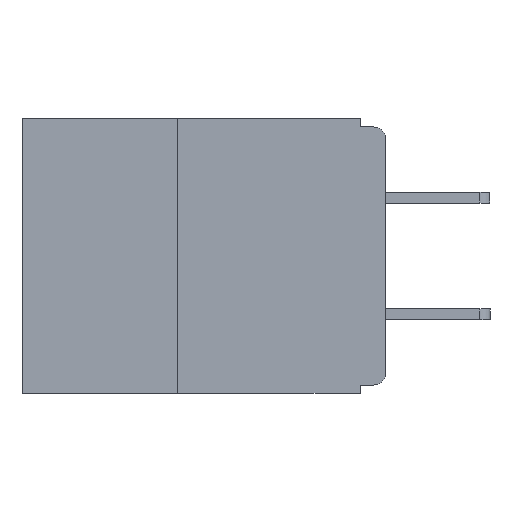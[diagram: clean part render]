
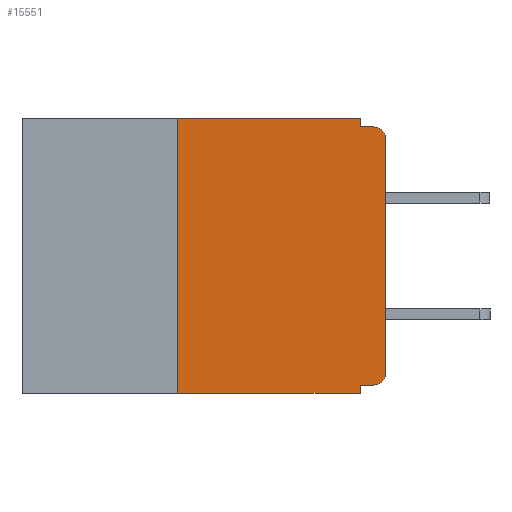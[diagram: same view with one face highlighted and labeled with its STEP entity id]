
A CAD part, left-side view. The second image highlights one B-rep face of the part: STEP entity #15551.
In plain terms, the highlighted planar face has unit normal (-1, 0, 0).
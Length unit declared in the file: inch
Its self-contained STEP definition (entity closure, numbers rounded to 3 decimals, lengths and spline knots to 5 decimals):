
#156 = LINE ( 'NONE', #7414, #13391 ) ;
#546 = CARTESIAN_POINT ( 'NONE',  ( 0., 0.437, 0. ) ) ;
#576 = ORIENTED_EDGE ( 'NONE', *, *, #13865, .F. ) ;
#692 = DIRECTION ( 'NONE',  ( 0., -1., 0. ) ) ;
#1141 = CARTESIAN_POINT ( 'NONE',  ( 0., 0.437, -0.33 ) ) ;
#1366 = CARTESIAN_POINT ( 'NONE',  ( 0., 0.031, 0. ) ) ;
#1687 = CARTESIAN_POINT ( 'NONE',  ( 0., 0.031, 0. ) ) ;
#1850 = VERTEX_POINT ( 'NONE', #1687 ) ;
#1886 = DIRECTION ( 'NONE',  ( 1., 0., 0. ) ) ;
#2242 = EDGE_CURVE ( 'NONE', #14894, #14790, #11142, .T. ) ;
#2300 = DIRECTION ( 'NONE',  ( 0., 0., 1. ) ) ;
#2543 = AXIS2_PLACEMENT_3D ( 'NONE', #3014, #3001, #2996 ) ;
#2635 = VERTEX_POINT ( 'NONE', #13340 ) ;
#2672 = CARTESIAN_POINT ( 'NONE',  ( 0., 0.015, -0.01 ) ) ;
#2711 = LINE ( 'NONE', #8479, #3135 ) ;
#2727 = VECTOR ( 'NONE', #15027, 39.37008 ) ;
#2996 = DIRECTION ( 'NONE',  ( 0., 0., -1. ) ) ;
#3001 = DIRECTION ( 'NONE',  ( -1., 0., 0. ) ) ;
#3014 = CARTESIAN_POINT ( 'NONE',  ( 0., 0.015, -0.025 ) ) ;
#3135 = VECTOR ( 'NONE', #3293, 39.37008 ) ;
#3293 = DIRECTION ( 'NONE',  ( 0., -1., 0. ) ) ;
#3350 = AXIS2_PLACEMENT_3D ( 'NONE', #13615, #15105, #15219 ) ;
#3510 = VECTOR ( 'NONE', #13485, 39.37008 ) ;
#4034 = AXIS2_PLACEMENT_3D ( 'NONE', #546, #1886, #10865 ) ;
#4115 = DIRECTION ( 'NONE',  ( 0., 0., -1. ) ) ;
#4569 = CIRCLE ( 'NONE', #2543, 0.015 ) ;
#5411 = EDGE_CURVE ( 'NONE', #15789, #10457, #12205, .T. ) ;
#5886 = LINE ( 'NONE', #14158, #15485 ) ;
#6221 = CARTESIAN_POINT ( 'NONE',  ( 0., 0.031, -0.33 ) ) ;
#6424 = CARTESIAN_POINT ( 'NONE',  ( 0., 0., -0.305 ) ) ;
#6653 = CARTESIAN_POINT ( 'NONE',  ( 0., 0.015, -0.32 ) ) ;
#6882 = LINE ( 'NONE', #10980, #3510 ) ;
#7287 = ORIENTED_EDGE ( 'NONE', *, *, #5411, .T. ) ;
#7289 = VECTOR ( 'NONE', #7389, 39.37008 ) ;
#7389 = DIRECTION ( 'NONE',  ( 0., 1., 0. ) ) ;
#7414 = CARTESIAN_POINT ( 'NONE',  ( 0., 0.25, -0.33 ) ) ;
#8040 = ORIENTED_EDGE ( 'NONE', *, *, #8428, .T. ) ;
#8296 = PLANE ( 'NONE',  #4034 ) ;
#8381 = CARTESIAN_POINT ( 'NONE',  ( 0., 0.031, -0.01 ) ) ;
#8394 = ORIENTED_EDGE ( 'NONE', *, *, #11517, .F. ) ;
#8428 = EDGE_CURVE ( 'NONE', #10171, #8513, #4569, .T. ) ;
#8479 = CARTESIAN_POINT ( 'NONE',  ( 0., 0.437, 0. ) ) ;
#8513 = VERTEX_POINT ( 'NONE', #2672 ) ;
#8784 = CARTESIAN_POINT ( 'NONE',  ( 0., 0., 0. ) ) ;
#8802 = EDGE_CURVE ( 'NONE', #1850, #9108, #15712, .T. ) ;
#8861 = CARTESIAN_POINT ( 'NONE',  ( 0., 0.25, -0.33 ) ) ;
#9108 = VERTEX_POINT ( 'NONE', #8381 ) ;
#9187 = EDGE_CURVE ( 'NONE', #14790, #10171, #12879, .T. ) ;
#9677 = EDGE_CURVE ( 'NONE', #15956, #1850, #2711, .T. ) ;
#10171 = VERTEX_POINT ( 'NONE', #14426 ) ;
#10397 = EDGE_CURVE ( 'NONE', #14894, #2635, #13982, .T. ) ;
#10457 = VERTEX_POINT ( 'NONE', #6221 ) ;
#10865 = DIRECTION ( 'NONE',  ( 0., 0., -1. ) ) ;
#10980 = CARTESIAN_POINT ( 'NONE',  ( 0., 0., -0.01 ) ) ;
#11142 = CIRCLE ( 'NONE', #3350, 0.015 ) ;
#11230 = FACE_OUTER_BOUND ( 'NONE', #11752, .T. ) ;
#11517 = EDGE_CURVE ( 'NONE', #9108, #8513, #6882, .T. ) ;
#11534 = ORIENTED_EDGE ( 'NONE', *, *, #11734, .F. ) ;
#11734 = EDGE_CURVE ( 'NONE', #15789, #15956, #156, .T. ) ;
#11752 = EDGE_LOOP ( 'NONE', ( #15307, #8040, #8394, #15761, #15446, #11534, #7287, #576, #14640, #11879 ) ) ;
#11879 = ORIENTED_EDGE ( 'NONE', *, *, #2242, .T. ) ;
#12205 = LINE ( 'NONE', #1141, #15065 ) ;
#12879 = LINE ( 'NONE', #8784, #2727 ) ;
#13340 = CARTESIAN_POINT ( 'NONE',  ( 0., 0.031, -0.32 ) ) ;
#13391 = VECTOR ( 'NONE', #2300, 39.37008 ) ;
#13485 = DIRECTION ( 'NONE',  ( 0., -1., 0. ) ) ;
#13615 = CARTESIAN_POINT ( 'NONE',  ( 0., 0.015, -0.305 ) ) ;
#13681 = CARTESIAN_POINT ( 'NONE',  ( 0., 0., -0.32 ) ) ;
#13865 = EDGE_CURVE ( 'NONE', #2635, #10457, #5886, .T. ) ;
#13982 = LINE ( 'NONE', #13681, #7289 ) ;
#14033 = DIRECTION ( 'NONE',  ( 0., 0., -1. ) ) ;
#14149 = CARTESIAN_POINT ( 'NONE',  ( 0., 0.25, 0. ) ) ;
#14158 = CARTESIAN_POINT ( 'NONE',  ( 0., 0.031, -0.33 ) ) ;
#14426 = CARTESIAN_POINT ( 'NONE',  ( 0., 0., -0.025 ) ) ;
#14640 = ORIENTED_EDGE ( 'NONE', *, *, #10397, .F. ) ;
#14790 = VERTEX_POINT ( 'NONE', #6424 ) ;
#14894 = VERTEX_POINT ( 'NONE', #6653 ) ;
#15027 = DIRECTION ( 'NONE',  ( 0., 0., 1. ) ) ;
#15065 = VECTOR ( 'NONE', #692, 39.37008 ) ;
#15105 = DIRECTION ( 'NONE',  ( -1., 0., 0. ) ) ;
#15219 = DIRECTION ( 'NONE',  ( 0., 0., -1. ) ) ;
#15307 = ORIENTED_EDGE ( 'NONE', *, *, #9187, .T. ) ;
#15351 = VECTOR ( 'NONE', #14033, 39.37008 ) ;
#15446 = ORIENTED_EDGE ( 'NONE', *, *, #9677, .F. ) ;
#15485 = VECTOR ( 'NONE', #4115, 39.37008 ) ;
#15551 = ADVANCED_FACE ( 'NONE', ( #11230 ), #8296, .F. ) ;
#15712 = LINE ( 'NONE', #1366, #15351 ) ;
#15761 = ORIENTED_EDGE ( 'NONE', *, *, #8802, .F. ) ;
#15789 = VERTEX_POINT ( 'NONE', #8861 ) ;
#15956 = VERTEX_POINT ( 'NONE', #14149 ) ;
